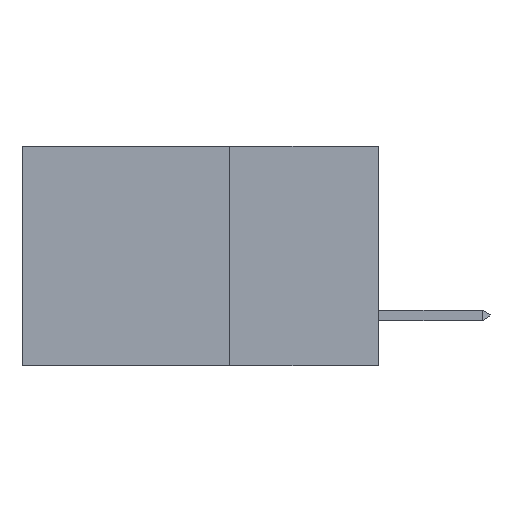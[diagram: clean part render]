
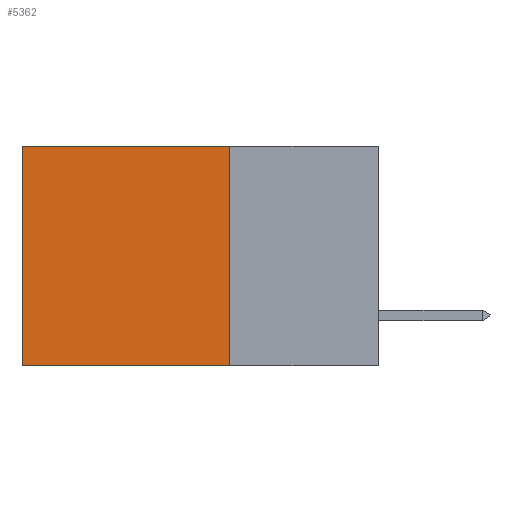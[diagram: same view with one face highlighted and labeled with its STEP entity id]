
A CAD part, left-side view. The second image highlights one B-rep face of the part: STEP entity #5362.
In plain terms, the highlighted planar face has unit normal (-1, 0, 0).
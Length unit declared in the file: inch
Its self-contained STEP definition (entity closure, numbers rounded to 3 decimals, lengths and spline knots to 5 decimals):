
#166 = LINE ( 'NONE', #6378, #4534 ) ;
#424 = LINE ( 'NONE', #2346, #7485 ) ;
#523 = VERTEX_POINT ( 'NONE', #6990 ) ;
#1071 = ORIENTED_EDGE ( 'NONE', *, *, #5379, .F. ) ;
#1383 = DIRECTION ( 'NONE',  ( 0., 0., -1. ) ) ;
#1987 = CARTESIAN_POINT ( 'NONE',  ( 0.2615, 0.25, 0. ) ) ;
#2238 = CARTESIAN_POINT ( 'NONE',  ( 0.2615, 0.25, -0.37 ) ) ;
#2346 = CARTESIAN_POINT ( 'NONE',  ( 0.2615, 0.6, -0.37 ) ) ;
#2392 = VECTOR ( 'NONE', #7320, 39.37008 ) ;
#3278 = DIRECTION ( 'NONE',  ( 1., 0., 0. ) ) ;
#4303 = DIRECTION ( 'NONE',  ( 0., 1., 0. ) ) ;
#4521 = EDGE_CURVE ( 'NONE', #6622, #10861, #4621, .T. ) ;
#4534 = VECTOR ( 'NONE', #4303, 39.37008 ) ;
#4621 = LINE ( 'NONE', #11897, #11297 ) ;
#5362 = ADVANCED_FACE ( 'NONE', ( #8677 ), #9874, .F. ) ;
#5379 = EDGE_CURVE ( 'NONE', #10861, #11954, #166, .T. ) ;
#5540 = DIRECTION ( 'NONE',  ( 0., 0., -1. ) ) ;
#5626 = AXIS2_PLACEMENT_3D ( 'NONE', #2238, #3278, #5540 ) ;
#6064 = LINE ( 'NONE', #1987, #2392 ) ;
#6378 = CARTESIAN_POINT ( 'NONE',  ( 0.2615, 0.25, -0.37 ) ) ;
#6622 = VERTEX_POINT ( 'NONE', #13085 ) ;
#6990 = CARTESIAN_POINT ( 'NONE',  ( 0.2615, 0.6, 0. ) ) ;
#7320 = DIRECTION ( 'NONE',  ( 0., 1., 0. ) ) ;
#7485 = VECTOR ( 'NONE', #1383, 39.37008 ) ;
#8677 = FACE_OUTER_BOUND ( 'NONE', #11239, .T. ) ;
#8705 = ORIENTED_EDGE ( 'NONE', *, *, #4521, .F. ) ;
#9874 = PLANE ( 'NONE',  #5626 ) ;
#10861 = VERTEX_POINT ( 'NONE', #12758 ) ;
#10894 = DIRECTION ( 'NONE',  ( 0., 0., -1. ) ) ;
#10968 = EDGE_CURVE ( 'NONE', #6622, #523, #6064, .T. ) ;
#11126 = EDGE_CURVE ( 'NONE', #523, #11954, #424, .T. ) ;
#11239 = EDGE_LOOP ( 'NONE', ( #12010, #1071, #8705, #11248 ) ) ;
#11248 = ORIENTED_EDGE ( 'NONE', *, *, #10968, .T. ) ;
#11257 = CARTESIAN_POINT ( 'NONE',  ( 0.2615, 0.6, -0.37 ) ) ;
#11297 = VECTOR ( 'NONE', #10894, 39.37008 ) ;
#11897 = CARTESIAN_POINT ( 'NONE',  ( 0.2615, 0.25, -0.37 ) ) ;
#11954 = VERTEX_POINT ( 'NONE', #11257 ) ;
#12010 = ORIENTED_EDGE ( 'NONE', *, *, #11126, .T. ) ;
#12758 = CARTESIAN_POINT ( 'NONE',  ( 0.2615, 0.25, -0.37 ) ) ;
#13085 = CARTESIAN_POINT ( 'NONE',  ( 0.2615, 0.25, 0. ) ) ;
